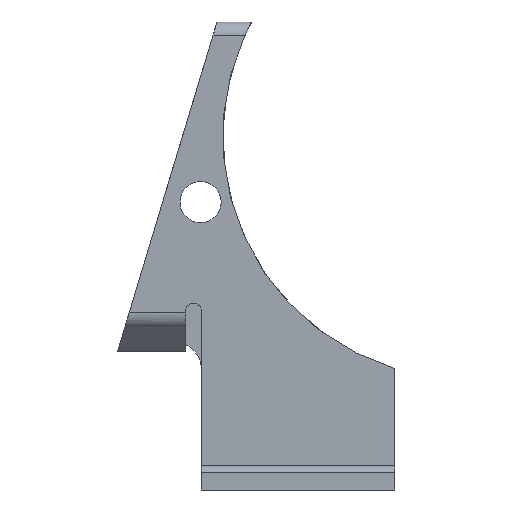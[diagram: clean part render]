
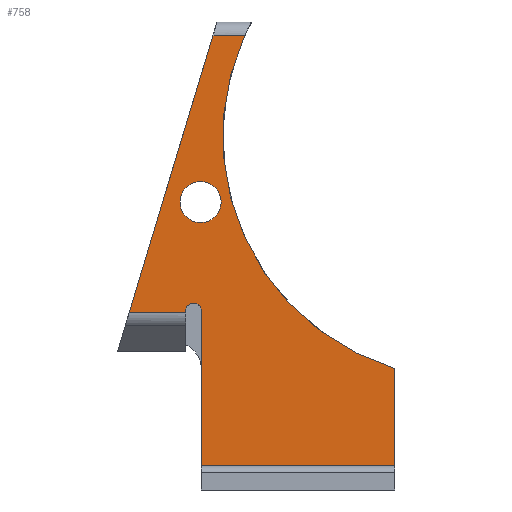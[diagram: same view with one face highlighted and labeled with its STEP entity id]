
A CAD part, left-side view. The second image highlights one B-rep face of the part: STEP entity #758.
In plain terms, the highlighted planar face has unit normal (-1, 0, 0).
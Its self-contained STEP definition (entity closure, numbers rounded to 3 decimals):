
#19=FACE_BOUND('',#98,.T.);
#24=PLANE('',#820);
#57=FACE_OUTER_BOUND('',#97,.T.);
#97=EDGE_LOOP('',(#528,#529,#530,#531,#532,#533,#534,#535,#536,#537,#538));
#98=EDGE_LOOP('',(#539));
#144=LINE('',#1139,#222);
#145=LINE('',#1142,#223);
#146=LINE('',#1146,#224);
#147=LINE('',#1150,#225);
#148=LINE('',#1152,#226);
#149=LINE('',#1154,#227);
#150=LINE('',#1158,#228);
#151=LINE('',#1159,#229);
#222=VECTOR('',#915,10.);
#223=VECTOR('',#918,10.);
#224=VECTOR('',#921,10.);
#225=VECTOR('',#924,10.);
#226=VECTOR('',#925,10.);
#227=VECTOR('',#926,10.);
#228=VECTOR('',#929,10.);
#229=VECTOR('',#930,10.);
#293=CIRCLE('',#809,1.525);
#298=CIRCLE('',#821,0.5);
#299=CIRCLE('',#822,0.5);
#300=CIRCLE('',#823,17.951);
#319=VERTEX_POINT('',#1107);
#329=VERTEX_POINT('',#1133);
#331=VERTEX_POINT('',#1137);
#332=VERTEX_POINT('',#1141);
#333=VERTEX_POINT('',#1143);
#334=VERTEX_POINT('',#1145);
#335=VERTEX_POINT('',#1147);
#336=VERTEX_POINT('',#1149);
#337=VERTEX_POINT('',#1151);
#338=VERTEX_POINT('',#1153);
#339=VERTEX_POINT('',#1155);
#340=VERTEX_POINT('',#1157);
#396=EDGE_CURVE('',#319,#319,#293,.T.);
#410=EDGE_CURVE('',#329,#331,#144,.T.);
#411=EDGE_CURVE('',#331,#332,#145,.T.);
#412=EDGE_CURVE('',#333,#332,#298,.T.);
#413=EDGE_CURVE('',#333,#334,#146,.T.);
#414=EDGE_CURVE('',#335,#334,#299,.T.);
#415=EDGE_CURVE('',#335,#336,#147,.T.);
#416=EDGE_CURVE('',#337,#336,#148,.T.);
#417=EDGE_CURVE('',#338,#337,#149,.T.);
#418=EDGE_CURVE('',#338,#339,#300,.T.);
#419=EDGE_CURVE('',#340,#339,#150,.T.);
#420=EDGE_CURVE('',#340,#329,#151,.T.);
#528=ORIENTED_EDGE('',*,*,#410,.T.);
#529=ORIENTED_EDGE('',*,*,#411,.T.);
#530=ORIENTED_EDGE('',*,*,#412,.F.);
#531=ORIENTED_EDGE('',*,*,#413,.T.);
#532=ORIENTED_EDGE('',*,*,#414,.F.);
#533=ORIENTED_EDGE('',*,*,#415,.T.);
#534=ORIENTED_EDGE('',*,*,#416,.F.);
#535=ORIENTED_EDGE('',*,*,#417,.F.);
#536=ORIENTED_EDGE('',*,*,#418,.T.);
#537=ORIENTED_EDGE('',*,*,#419,.F.);
#538=ORIENTED_EDGE('',*,*,#420,.T.);
#539=ORIENTED_EDGE('',*,*,#396,.T.);
#758=ADVANCED_FACE('',(#57,#19),#24,.T.);
#809=AXIS2_PLACEMENT_3D('',#1109,#886,#887);
#820=AXIS2_PLACEMENT_3D('',#1140,#916,#917);
#821=AXIS2_PLACEMENT_3D('',#1144,#919,#920);
#822=AXIS2_PLACEMENT_3D('',#1148,#922,#923);
#823=AXIS2_PLACEMENT_3D('',#1156,#927,#928);
#886=DIRECTION('center_axis',(1.,0.,0.));
#887=DIRECTION('ref_axis',(0.,1.,0.));
#915=DIRECTION('',(0.,-1.,0.));
#916=DIRECTION('center_axis',(-1.,0.,0.));
#917=DIRECTION('ref_axis',(0.,0.,1.));
#918=DIRECTION('',(0.,0.,1.));
#919=DIRECTION('center_axis',(-1.,0.,0.));
#920=DIRECTION('ref_axis',(0.,0.707,0.707));
#921=DIRECTION('',(0.,-1.,0.));
#922=DIRECTION('center_axis',(-1.,0.,0.));
#923=DIRECTION('ref_axis',(0.,-0.707,0.707));
#924=DIRECTION('',(0.,0.,-1.));
#925=DIRECTION('',(0.,1.,0.));
#926=DIRECTION('',(0.,0.,-1.));
#927=DIRECTION('center_axis',(1.,0.,0.));
#928=DIRECTION('ref_axis',(0.,-1.,0.));
#929=DIRECTION('',(0.,-1.,0.));
#930=DIRECTION('',(0.,0.289,-0.957));
#1107=CARTESIAN_POINT('',(-6.925,12.833,-12.038));
#1109=CARTESIAN_POINT('Origin',(-6.925,14.358,-12.038));
#1133=CARTESIAN_POINT('',(-6.925,19.645,-20.231));
#1137=CARTESIAN_POINT('',(-6.925,15.45,-20.231));
#1139=CARTESIAN_POINT('',(-6.925,15.45,-20.231));
#1140=CARTESIAN_POINT('Origin',(-6.925,0.,-32.05));
#1141=CARTESIAN_POINT('',(-6.925,15.45,-20.04));
#1142=CARTESIAN_POINT('',(-6.925,15.45,-27.225));
#1143=CARTESIAN_POINT('',(-6.925,14.95,-19.54));
#1144=CARTESIAN_POINT('Origin',(-6.925,14.95,-20.04));
#1145=CARTESIAN_POINT('',(-6.925,14.8,-19.54));
#1146=CARTESIAN_POINT('',(-6.925,7.725,-19.54));
#1147=CARTESIAN_POINT('',(-6.925,14.3,-20.04));
#1148=CARTESIAN_POINT('Origin',(-6.925,14.8,-20.04));
#1149=CARTESIAN_POINT('',(-6.925,14.3,-31.55));
#1150=CARTESIAN_POINT('',(-6.925,14.3,-27.225));
#1151=CARTESIAN_POINT('',(-6.925,0.,-31.55));
#1152=CARTESIAN_POINT('',(-6.925,0.,-31.55));
#1153=CARTESIAN_POINT('',(-6.925,0.,-24.35));
#1154=CARTESIAN_POINT('',(-6.925,0.,1.3));
#1155=CARTESIAN_POINT('',(-6.925,11.086,0.3));
#1156=CARTESIAN_POINT('Origin',(-6.925,-5.234,-7.178));
#1157=CARTESIAN_POINT('',(-6.925,13.442,0.3));
#1158=CARTESIAN_POINT('',(-6.925,0.,0.3));
#1159=CARTESIAN_POINT('',(-6.925,17.207,-12.161));
